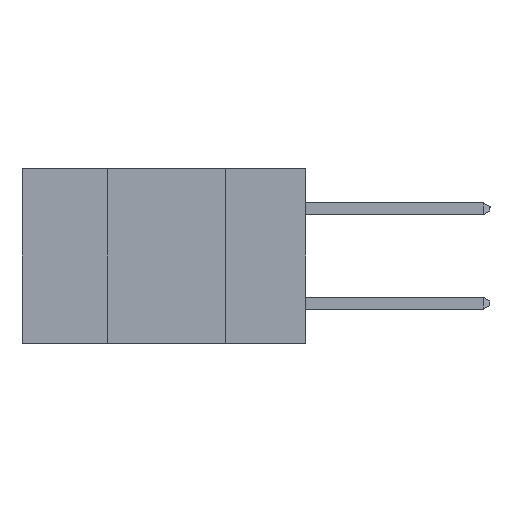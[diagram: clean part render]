
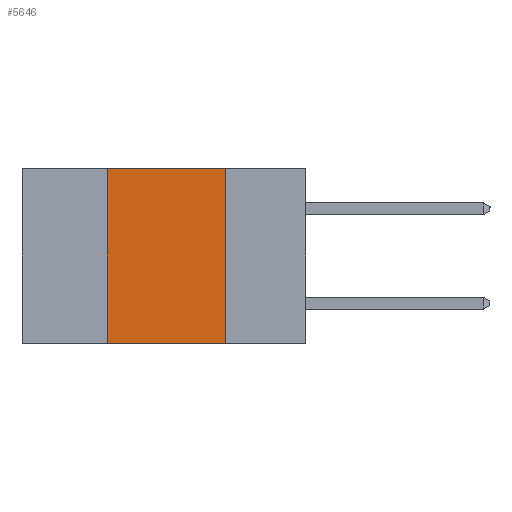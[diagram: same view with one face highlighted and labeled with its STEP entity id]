
A CAD part, left-side view. The second image highlights one B-rep face of the part: STEP entity #5646.
In plain terms, the highlighted planar face has unit normal (-1, 0, 0).
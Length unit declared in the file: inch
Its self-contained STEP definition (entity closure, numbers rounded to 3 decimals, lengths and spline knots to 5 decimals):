
#307 = CARTESIAN_POINT ( 'NONE',  ( 0., 0.17, -0.37 ) ) ;
#322 = ORIENTED_EDGE ( 'NONE', *, *, #7494, .F. ) ;
#693 = ORIENTED_EDGE ( 'NONE', *, *, #8946, .T. ) ;
#856 = VECTOR ( 'NONE', #7380, 39.37008 ) ;
#1220 = VECTOR ( 'NONE', #5881, 39.37008 ) ;
#1254 = LINE ( 'NONE', #5259, #1220 ) ;
#2730 = CARTESIAN_POINT ( 'NONE',  ( 0., 0.42, -0.37 ) ) ;
#3357 = VECTOR ( 'NONE', #8399, 39.37008 ) ;
#3964 = ORIENTED_EDGE ( 'NONE', *, *, #10138, .F. ) ;
#4184 = EDGE_LOOP ( 'NONE', ( #3964, #7575, #322, #693 ) ) ;
#4312 = VERTEX_POINT ( 'NONE', #7301 ) ;
#4431 = CARTESIAN_POINT ( 'NONE',  ( 0., 0.42, 0. ) ) ;
#4917 = FACE_OUTER_BOUND ( 'NONE', #4184, .T. ) ;
#4980 = VERTEX_POINT ( 'NONE', #4431 ) ;
#5066 = VECTOR ( 'NONE', #5318, 39.37008 ) ;
#5155 = CARTESIAN_POINT ( 'NONE',  ( 0., 0.42, -0.37 ) ) ;
#5259 = CARTESIAN_POINT ( 'NONE',  ( 0., 0.6, 0. ) ) ;
#5318 = DIRECTION ( 'NONE',  ( 0., -1., 0. ) ) ;
#5646 = ADVANCED_FACE ( 'NONE', ( #4917 ), #7132, .F. ) ;
#5881 = DIRECTION ( 'NONE',  ( 0., -1., 0. ) ) ;
#6089 = CARTESIAN_POINT ( 'NONE',  ( 0., 0.6, -0.37 ) ) ;
#6565 = CARTESIAN_POINT ( 'NONE',  ( 0., 0.6, 0. ) ) ;
#7132 = PLANE ( 'NONE',  #8552 ) ;
#7179 = VERTEX_POINT ( 'NONE', #9103 ) ;
#7288 = DIRECTION ( 'NONE',  ( 1., 0., 0. ) ) ;
#7301 = CARTESIAN_POINT ( 'NONE',  ( 0., 0.17, 0. ) ) ;
#7380 = DIRECTION ( 'NONE',  ( 0., 0., 1. ) ) ;
#7494 = EDGE_CURVE ( 'NONE', #9379, #4980, #8263, .T. ) ;
#7575 = ORIENTED_EDGE ( 'NONE', *, *, #9789, .F. ) ;
#8263 = LINE ( 'NONE', #5155, #856 ) ;
#8399 = DIRECTION ( 'NONE',  ( 0., 0., -1. ) ) ;
#8552 = AXIS2_PLACEMENT_3D ( 'NONE', #6565, #7288, #8735 ) ;
#8735 = DIRECTION ( 'NONE',  ( 0., 0., -1. ) ) ;
#8946 = EDGE_CURVE ( 'NONE', #9379, #7179, #9968, .T. ) ;
#9103 = CARTESIAN_POINT ( 'NONE',  ( 0., 0.17, -0.37 ) ) ;
#9219 = LINE ( 'NONE', #307, #3357 ) ;
#9379 = VERTEX_POINT ( 'NONE', #2730 ) ;
#9789 = EDGE_CURVE ( 'NONE', #4980, #4312, #1254, .T. ) ;
#9968 = LINE ( 'NONE', #6089, #5066 ) ;
#10138 = EDGE_CURVE ( 'NONE', #4312, #7179, #9219, .T. ) ;
